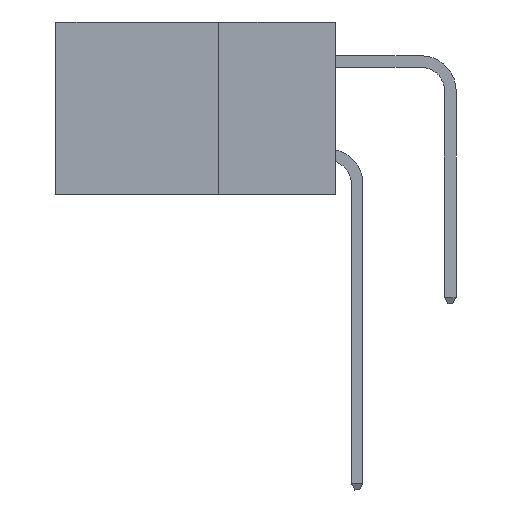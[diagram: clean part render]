
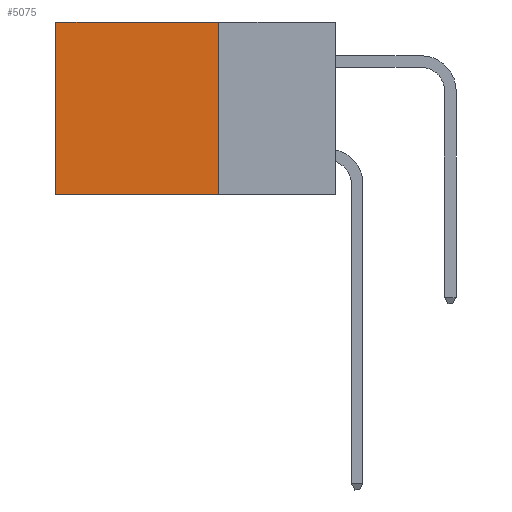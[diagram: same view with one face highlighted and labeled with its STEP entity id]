
A CAD part, left-side view. The second image highlights one B-rep face of the part: STEP entity #5075.
In plain terms, the highlighted planar face has unit normal (-1, 0, 0).
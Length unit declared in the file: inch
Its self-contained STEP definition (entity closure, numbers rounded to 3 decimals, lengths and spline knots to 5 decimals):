
#833 = EDGE_CURVE ( 'NONE', #6838, #14632, #11388, .T. ) ;
#913 = EDGE_CURVE ( 'NONE', #10833, #1975, #3800, .T. ) ;
#975 = ORIENTED_EDGE ( 'NONE', *, *, #833, .T. ) ;
#1248 = DIRECTION ( 'NONE',  ( 0., 1., 0. ) ) ;
#1696 = CARTESIAN_POINT ( 'NONE',  ( 0.2875, 0.25, -0.37 ) ) ;
#1717 = CARTESIAN_POINT ( 'NONE',  ( 0.2875, 0.25, 0. ) ) ;
#1975 = VERTEX_POINT ( 'NONE', #20552 ) ;
#2183 = CARTESIAN_POINT ( 'NONE',  ( 0.2875, 0.25, 0. ) ) ;
#3800 = LINE ( 'NONE', #22188, #11031 ) ;
#3922 = FACE_OUTER_BOUND ( 'NONE', #13527, .T. ) ;
#4242 = AXIS2_PLACEMENT_3D ( 'NONE', #1717, #16554, #22783 ) ;
#5075 = ADVANCED_FACE ( 'NONE', ( #3922 ), #12242, .F. ) ;
#5543 = EDGE_CURVE ( 'NONE', #6838, #10833, #20870, .T. ) ;
#6838 = VERTEX_POINT ( 'NONE', #24105 ) ;
#6905 = ORIENTED_EDGE ( 'NONE', *, *, #913, .F. ) ;
#10833 = VERTEX_POINT ( 'NONE', #1696 ) ;
#11031 = VECTOR ( 'NONE', #1248, 39.37008 ) ;
#11388 = LINE ( 'NONE', #2183, #27397 ) ;
#12242 = PLANE ( 'NONE',  #4242 ) ;
#12496 = VECTOR ( 'NONE', #16243, 39.37008 ) ;
#13527 = EDGE_LOOP ( 'NONE', ( #14540, #6905, #19508, #975 ) ) ;
#14540 = ORIENTED_EDGE ( 'NONE', *, *, #18596, .T. ) ;
#14632 = VERTEX_POINT ( 'NONE', #24587 ) ;
#15984 = LINE ( 'NONE', #19854, #22642 ) ;
#16243 = DIRECTION ( 'NONE',  ( 0., 0., -1. ) ) ;
#16554 = DIRECTION ( 'NONE',  ( 1., 0., 0. ) ) ;
#18596 = EDGE_CURVE ( 'NONE', #14632, #1975, #15984, .T. ) ;
#19508 = ORIENTED_EDGE ( 'NONE', *, *, #5543, .F. ) ;
#19854 = CARTESIAN_POINT ( 'NONE',  ( 0.2875, 0.6, 0. ) ) ;
#19895 = CARTESIAN_POINT ( 'NONE',  ( 0.2875, 0.25, 0. ) ) ;
#20552 = CARTESIAN_POINT ( 'NONE',  ( 0.2875, 0.6, -0.37 ) ) ;
#20870 = LINE ( 'NONE', #19895, #12496 ) ;
#22188 = CARTESIAN_POINT ( 'NONE',  ( 0.2875, 0.25, -0.37 ) ) ;
#22642 = VECTOR ( 'NONE', #26339, 39.37008 ) ;
#22783 = DIRECTION ( 'NONE',  ( 0., 0., -1. ) ) ;
#24105 = CARTESIAN_POINT ( 'NONE',  ( 0.2875, 0.25, 0. ) ) ;
#24587 = CARTESIAN_POINT ( 'NONE',  ( 0.2875, 0.6, 0. ) ) ;
#26028 = DIRECTION ( 'NONE',  ( 0., 1., 0. ) ) ;
#26339 = DIRECTION ( 'NONE',  ( 0., 0., -1. ) ) ;
#27397 = VECTOR ( 'NONE', #26028, 39.37008 ) ;
